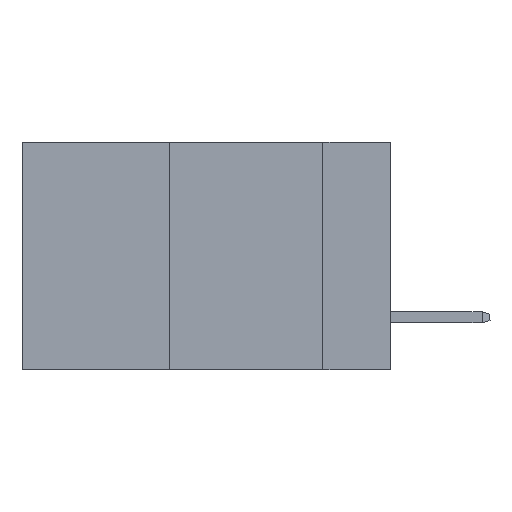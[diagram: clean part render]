
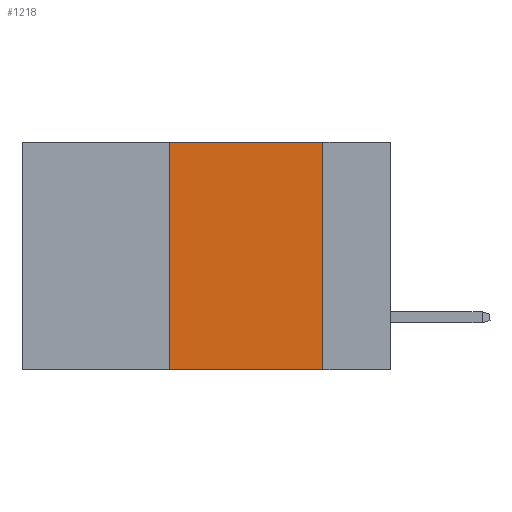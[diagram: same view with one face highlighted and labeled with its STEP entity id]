
A CAD part, left-side view. The second image highlights one B-rep face of the part: STEP entity #1218.
In plain terms, the highlighted planar face has unit normal (-1, 0, 0).
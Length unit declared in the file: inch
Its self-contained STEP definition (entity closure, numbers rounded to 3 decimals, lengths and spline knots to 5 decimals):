
#378 = CARTESIAN_POINT ( 'NONE',  ( 0., 0.11, -0.37 ) ) ;
#427 = EDGE_CURVE ( 'NONE', #6765, #596, #7529, .T. ) ;
#584 = CARTESIAN_POINT ( 'NONE',  ( 0., 0.11, 0. ) ) ;
#596 = VERTEX_POINT ( 'NONE', #4214 ) ;
#1050 = ORIENTED_EDGE ( 'NONE', *, *, #8616, .F. ) ;
#1218 = ADVANCED_FACE ( 'NONE', ( #8801 ), #7490, .F. ) ;
#1383 = ORIENTED_EDGE ( 'NONE', *, *, #2828, .T. ) ;
#1927 = EDGE_LOOP ( 'NONE', ( #1979, #1050, #3468, #1383 ) ) ;
#1979 = ORIENTED_EDGE ( 'NONE', *, *, #6889, .F. ) ;
#2045 = LINE ( 'NONE', #584, #4960 ) ;
#2312 = DIRECTION ( 'NONE',  ( 0., 0., 1. ) ) ;
#2456 = VECTOR ( 'NONE', #4740, 39.37008 ) ;
#2628 = CARTESIAN_POINT ( 'NONE',  ( 0., 0.6, 0. ) ) ;
#2678 = CARTESIAN_POINT ( 'NONE',  ( 0., 0.6, 0. ) ) ;
#2828 = EDGE_CURVE ( 'NONE', #6765, #3166, #4853, .T. ) ;
#3166 = VERTEX_POINT ( 'NONE', #378 ) ;
#3249 = DIRECTION ( 'NONE',  ( 1., 0., 0. ) ) ;
#3315 = DIRECTION ( 'NONE',  ( 0., 0., -1. ) ) ;
#3320 = DIRECTION ( 'NONE',  ( 0., 0., -1. ) ) ;
#3468 = ORIENTED_EDGE ( 'NONE', *, *, #427, .F. ) ;
#3908 = DIRECTION ( 'NONE',  ( 0., -1., 0. ) ) ;
#3947 = CARTESIAN_POINT ( 'NONE',  ( 0., 0.6, -0.37 ) ) ;
#4164 = VERTEX_POINT ( 'NONE', #8727 ) ;
#4214 = CARTESIAN_POINT ( 'NONE',  ( 0., 0.36, 0. ) ) ;
#4646 = VECTOR ( 'NONE', #3908, 39.37008 ) ;
#4740 = DIRECTION ( 'NONE',  ( 0., -1., 0. ) ) ;
#4853 = LINE ( 'NONE', #3947, #4646 ) ;
#4960 = VECTOR ( 'NONE', #3320, 39.37008 ) ;
#5339 = CARTESIAN_POINT ( 'NONE',  ( 0., 0.36, -0.37 ) ) ;
#5779 = CARTESIAN_POINT ( 'NONE',  ( 0., 0.36, 0. ) ) ;
#6765 = VERTEX_POINT ( 'NONE', #5339 ) ;
#6889 = EDGE_CURVE ( 'NONE', #4164, #3166, #2045, .T. ) ;
#7490 = PLANE ( 'NONE',  #7863 ) ;
#7529 = LINE ( 'NONE', #5779, #8708 ) ;
#7863 = AXIS2_PLACEMENT_3D ( 'NONE', #2628, #3249, #3315 ) ;
#8616 = EDGE_CURVE ( 'NONE', #596, #4164, #8962, .T. ) ;
#8708 = VECTOR ( 'NONE', #2312, 39.37008 ) ;
#8727 = CARTESIAN_POINT ( 'NONE',  ( 0., 0.11, 0. ) ) ;
#8801 = FACE_OUTER_BOUND ( 'NONE', #1927, .T. ) ;
#8962 = LINE ( 'NONE', #2678, #2456 ) ;
